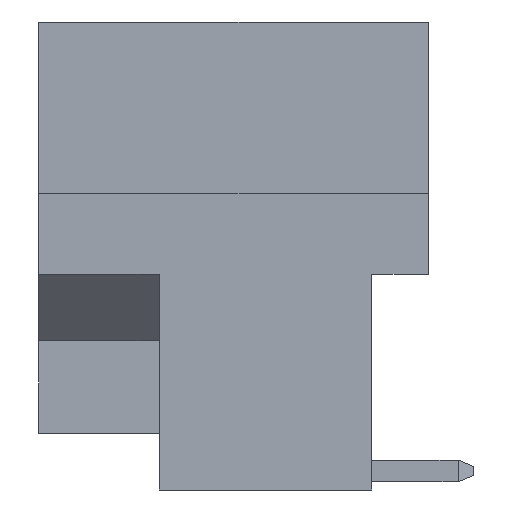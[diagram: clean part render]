
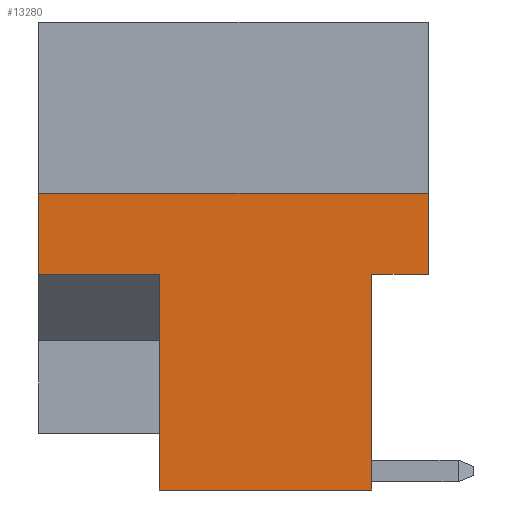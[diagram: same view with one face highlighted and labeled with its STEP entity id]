
A CAD part, left-side view. The second image highlights one B-rep face of the part: STEP entity #13280.
In plain terms, the highlighted planar face has unit normal (-1, 0, 0).
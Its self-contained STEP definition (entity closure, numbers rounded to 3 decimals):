
#1039 = VERTEX_POINT ( 'NONE', #7675 ) ;
#1563 = VECTOR ( 'NONE', #3876, 1000. ) ;
#1680 = DIRECTION ( 'NONE',  ( 0., 1., 0. ) ) ;
#1817 = VECTOR ( 'NONE', #11425, 1000. ) ;
#2357 = ORIENTED_EDGE ( 'NONE', *, *, #10199, .F. ) ;
#3009 = CARTESIAN_POINT ( 'NONE',  ( 0., 7.597, -13.2 ) ) ;
#3273 = LINE ( 'NONE', #12699, #11415 ) ;
#3280 = EDGE_CURVE ( 'NONE', #14782, #1039, #9096, .T. ) ;
#3566 = CARTESIAN_POINT ( 'NONE',  ( 0., 1.6, -13.2 ) ) ;
#3603 = PLANE ( 'NONE',  #5615 ) ;
#3876 = DIRECTION ( 'NONE',  ( 0., -1., 0. ) ) ;
#4112 = ORIENTED_EDGE ( 'NONE', *, *, #3280, .F. ) ;
#4453 = CARTESIAN_POINT ( 'NONE',  ( 0., 7.597, -13.2 ) ) ;
#5039 = ORIENTED_EDGE ( 'NONE', *, *, #10932, .F. ) ;
#5041 = CARTESIAN_POINT ( 'NONE',  ( 0., 10.998, -13.2 ) ) ;
#5615 = AXIS2_PLACEMENT_3D ( 'NONE', #15201, #9471, #10481 ) ;
#5946 = ORIENTED_EDGE ( 'NONE', *, *, #12320, .F. ) ;
#6892 = VERTEX_POINT ( 'NONE', #3009 ) ;
#7021 = VERTEX_POINT ( 'NONE', #10712 ) ;
#7022 = LINE ( 'NONE', #10412, #10172 ) ;
#7128 = ORIENTED_EDGE ( 'NONE', *, *, #12785, .T. ) ;
#7675 = CARTESIAN_POINT ( 'NONE',  ( 0., 10.998, -4.826 ) ) ;
#7833 = VECTOR ( 'NONE', #8071, 1000. ) ;
#7945 = LINE ( 'NONE', #14830, #12143 ) ;
#8013 = FACE_OUTER_BOUND ( 'NONE', #8144, .T. ) ;
#8069 = VERTEX_POINT ( 'NONE', #3566 ) ;
#8071 = DIRECTION ( 'NONE',  ( 0., 0., 1. ) ) ;
#8144 = EDGE_LOOP ( 'NONE', ( #5039, #2357, #7128, #5946, #4112, #10087, #8736, #12613 ) ) ;
#8321 = DIRECTION ( 'NONE',  ( 0., 1., 0. ) ) ;
#8534 = EDGE_CURVE ( 'NONE', #6892, #11946, #8924, .T. ) ;
#8736 = ORIENTED_EDGE ( 'NONE', *, *, #8534, .F. ) ;
#8820 = CARTESIAN_POINT ( 'NONE',  ( 0., 10.998, -7.112 ) ) ;
#8873 = DIRECTION ( 'NONE',  ( 0., 0., -1. ) ) ;
#8924 = LINE ( 'NONE', #4453, #7833 ) ;
#9096 = LINE ( 'NONE', #13815, #11058 ) ;
#9107 = LINE ( 'NONE', #11275, #1817 ) ;
#9471 = DIRECTION ( 'NONE',  ( 1., 0., 0. ) ) ;
#10087 = ORIENTED_EDGE ( 'NONE', *, *, #11695, .F. ) ;
#10172 = VECTOR ( 'NONE', #8321, 1000. ) ;
#10199 = EDGE_CURVE ( 'NONE', #7021, #13245, #3273, .T. ) ;
#10412 = CARTESIAN_POINT ( 'NONE',  ( 0., 7.597, -7.112 ) ) ;
#10463 = EDGE_CURVE ( 'NONE', #6892, #8069, #10986, .T. ) ;
#10481 = DIRECTION ( 'NONE',  ( 0., 0., -1. ) ) ;
#10712 = CARTESIAN_POINT ( 'NONE',  ( 0., 0., -7.112 ) ) ;
#10932 = EDGE_CURVE ( 'NONE', #13245, #8069, #7945, .T. ) ;
#10986 = LINE ( 'NONE', #5041, #1563 ) ;
#11058 = VECTOR ( 'NONE', #12655, 1000. ) ;
#11229 = DIRECTION ( 'NONE',  ( 0., -1., 0. ) ) ;
#11275 = CARTESIAN_POINT ( 'NONE',  ( 0., 0., 0. ) ) ;
#11415 = VECTOR ( 'NONE', #1680, 1000. ) ;
#11425 = DIRECTION ( 'NONE',  ( 0., 0., 1. ) ) ;
#11695 = EDGE_CURVE ( 'NONE', #11946, #14782, #7022, .T. ) ;
#11847 = VERTEX_POINT ( 'NONE', #14350 ) ;
#11865 = LINE ( 'NONE', #14335, #12415 ) ;
#11946 = VERTEX_POINT ( 'NONE', #13117 ) ;
#12143 = VECTOR ( 'NONE', #8873, 1000. ) ;
#12320 = EDGE_CURVE ( 'NONE', #1039, #11847, #11865, .T. ) ;
#12415 = VECTOR ( 'NONE', #11229, 1000. ) ;
#12613 = ORIENTED_EDGE ( 'NONE', *, *, #10463, .T. ) ;
#12655 = DIRECTION ( 'NONE',  ( 0., 0., 1. ) ) ;
#12699 = CARTESIAN_POINT ( 'NONE',  ( 0., 0., -7.112 ) ) ;
#12785 = EDGE_CURVE ( 'NONE', #7021, #11847, #9107, .T. ) ;
#13117 = CARTESIAN_POINT ( 'NONE',  ( 0., 7.597, -7.112 ) ) ;
#13245 = VERTEX_POINT ( 'NONE', #13728 ) ;
#13280 = ADVANCED_FACE ( 'NONE', ( #8013 ), #3603, .F. ) ;
#13728 = CARTESIAN_POINT ( 'NONE',  ( 0., 1.6, -7.112 ) ) ;
#13815 = CARTESIAN_POINT ( 'NONE',  ( 0., 10.998, 0. ) ) ;
#14335 = CARTESIAN_POINT ( 'NONE',  ( 0., 10.998, -4.826 ) ) ;
#14350 = CARTESIAN_POINT ( 'NONE',  ( 0., 0., -4.826 ) ) ;
#14782 = VERTEX_POINT ( 'NONE', #8820 ) ;
#14830 = CARTESIAN_POINT ( 'NONE',  ( 0., 1.6, 86.902 ) ) ;
#15201 = CARTESIAN_POINT ( 'NONE',  ( 0., 10.998, 0. ) ) ;
